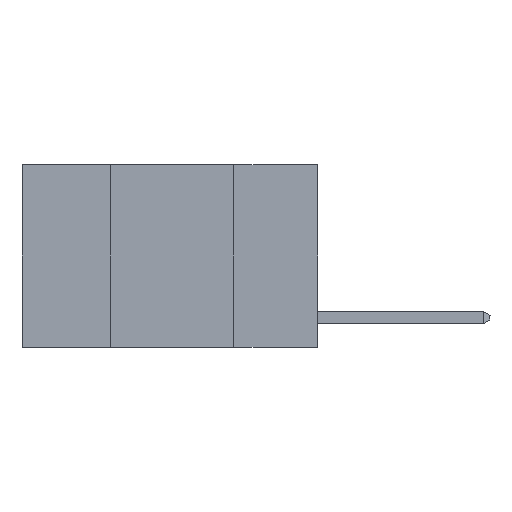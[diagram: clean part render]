
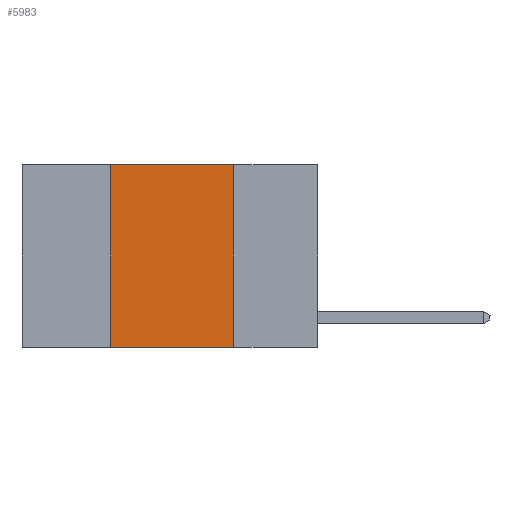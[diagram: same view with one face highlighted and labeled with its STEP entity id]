
A CAD part, left-side view. The second image highlights one B-rep face of the part: STEP entity #5983.
In plain terms, the highlighted planar face has unit normal (-1, 0, 0).
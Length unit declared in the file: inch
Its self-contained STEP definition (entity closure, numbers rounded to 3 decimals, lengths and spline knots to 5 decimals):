
#108 = CARTESIAN_POINT ( 'NONE',  ( 0., 0.6, -0.37 ) ) ;
#1945 = LINE ( 'NONE', #11333, #24721 ) ;
#3011 = VERTEX_POINT ( 'NONE', #10477 ) ;
#3405 = VECTOR ( 'NONE', #18094, 39.37008 ) ;
#5003 = VECTOR ( 'NONE', #18688, 39.37008 ) ;
#5337 = CARTESIAN_POINT ( 'NONE',  ( 0., 0.42, 0. ) ) ;
#5434 = EDGE_LOOP ( 'NONE', ( #10915, #23083, #6405, #9024 ) ) ;
#5983 = ADVANCED_FACE ( 'NONE', ( #17822 ), #23702, .F. ) ;
#6405 = ORIENTED_EDGE ( 'NONE', *, *, #18676, .F. ) ;
#8136 = VERTEX_POINT ( 'NONE', #15304 ) ;
#8204 = LINE ( 'NONE', #108, #5003 ) ;
#8233 = VERTEX_POINT ( 'NONE', #22668 ) ;
#9024 = ORIENTED_EDGE ( 'NONE', *, *, #20338, .T. ) ;
#9459 = CARTESIAN_POINT ( 'NONE',  ( 0., 0.17, -0.37 ) ) ;
#9500 = LINE ( 'NONE', #22636, #3405 ) ;
#9942 = DIRECTION ( 'NONE',  ( 0., 0., -1. ) ) ;
#10034 = DIRECTION ( 'NONE',  ( 1., 0., 0. ) ) ;
#10477 = CARTESIAN_POINT ( 'NONE',  ( 0., 0.42, -0.37 ) ) ;
#10915 = ORIENTED_EDGE ( 'NONE', *, *, #16302, .F. ) ;
#11333 = CARTESIAN_POINT ( 'NONE',  ( 0., 0.17, 0. ) ) ;
#13186 = VERTEX_POINT ( 'NONE', #9459 ) ;
#14637 = DIRECTION ( 'NONE',  ( 0., 0., 1. ) ) ;
#15304 = CARTESIAN_POINT ( 'NONE',  ( 0., 0.42, 0. ) ) ;
#16302 = EDGE_CURVE ( 'NONE', #8233, #13186, #1945, .T. ) ;
#17766 = LINE ( 'NONE', #5337, #28528 ) ;
#17822 = FACE_OUTER_BOUND ( 'NONE', #5434, .T. ) ;
#18094 = DIRECTION ( 'NONE',  ( 0., -1., 0. ) ) ;
#18676 = EDGE_CURVE ( 'NONE', #3011, #8136, #17766, .T. ) ;
#18688 = DIRECTION ( 'NONE',  ( 0., -1., 0. ) ) ;
#20338 = EDGE_CURVE ( 'NONE', #3011, #13186, #8204, .T. ) ;
#22636 = CARTESIAN_POINT ( 'NONE',  ( 0., 0.6, 0. ) ) ;
#22668 = CARTESIAN_POINT ( 'NONE',  ( 0., 0.17, 0. ) ) ;
#23059 = DIRECTION ( 'NONE',  ( 0., 0., -1. ) ) ;
#23083 = ORIENTED_EDGE ( 'NONE', *, *, #26667, .F. ) ;
#23702 = PLANE ( 'NONE',  #25724 ) ;
#23891 = CARTESIAN_POINT ( 'NONE',  ( 0., 0.6, 0. ) ) ;
#24721 = VECTOR ( 'NONE', #23059, 39.37008 ) ;
#25724 = AXIS2_PLACEMENT_3D ( 'NONE', #23891, #10034, #9942 ) ;
#26667 = EDGE_CURVE ( 'NONE', #8136, #8233, #9500, .T. ) ;
#28528 = VECTOR ( 'NONE', #14637, 39.37008 ) ;
